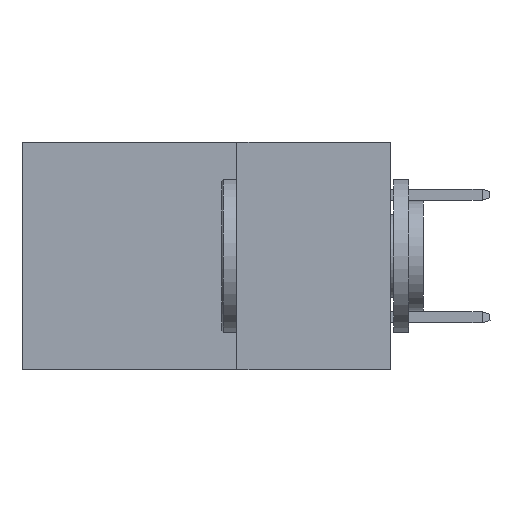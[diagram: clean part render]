
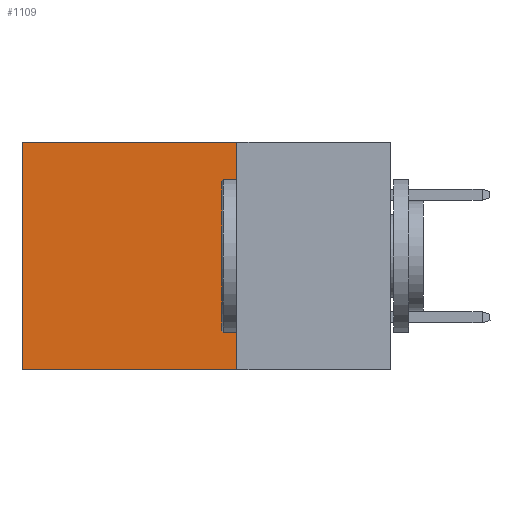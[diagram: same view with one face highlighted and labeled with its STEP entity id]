
A CAD part, left-side view. The second image highlights one B-rep face of the part: STEP entity #1109.
In plain terms, the highlighted planar face has unit normal (-1, 0, 0).
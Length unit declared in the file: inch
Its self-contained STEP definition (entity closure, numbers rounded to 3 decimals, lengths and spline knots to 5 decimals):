
#375 = EDGE_CURVE ( 'NONE', #5751, #5305, #4134, .T. ) ;
#1109 = ADVANCED_FACE ( 'NONE', ( #7847 ), #7928, .F. ) ;
#1123 = DIRECTION ( 'NONE',  ( 0., 0., -1. ) ) ;
#1485 = LINE ( 'NONE', #7017, #2935 ) ;
#1949 = ORIENTED_EDGE ( 'NONE', *, *, #10563, .F. ) ;
#2291 = LINE ( 'NONE', #9140, #10868 ) ;
#2491 = DIRECTION ( 'NONE',  ( 0., 1., 0. ) ) ;
#2551 = VECTOR ( 'NONE', #2491, 39.37008 ) ;
#2935 = VECTOR ( 'NONE', #5424, 39.37008 ) ;
#3433 = AXIS2_PLACEMENT_3D ( 'NONE', #3686, #5379, #1123 ) ;
#3471 = VERTEX_POINT ( 'NONE', #6926 ) ;
#3686 = CARTESIAN_POINT ( 'NONE',  ( 0.2875, 0.25, 0. ) ) ;
#4134 = LINE ( 'NONE', #4436, #5934 ) ;
#4308 = CARTESIAN_POINT ( 'NONE',  ( 0.2875, 0.25, -0.37 ) ) ;
#4430 = ORIENTED_EDGE ( 'NONE', *, *, #9543, .F. ) ;
#4436 = CARTESIAN_POINT ( 'NONE',  ( 0.2875, 0.25, 0. ) ) ;
#5018 = CARTESIAN_POINT ( 'NONE',  ( 0.2875, 0.6, -0.37 ) ) ;
#5305 = VERTEX_POINT ( 'NONE', #8914 ) ;
#5379 = DIRECTION ( 'NONE',  ( 1., 0., 0. ) ) ;
#5424 = DIRECTION ( 'NONE',  ( 0., 0., -1. ) ) ;
#5751 = VERTEX_POINT ( 'NONE', #9515 ) ;
#5788 = ORIENTED_EDGE ( 'NONE', *, *, #9982, .T. ) ;
#5934 = VECTOR ( 'NONE', #10287, 39.37008 ) ;
#6057 = EDGE_LOOP ( 'NONE', ( #5788, #1949, #4430, #7060 ) ) ;
#6926 = CARTESIAN_POINT ( 'NONE',  ( 0.2875, 0.25, -0.37 ) ) ;
#7017 = CARTESIAN_POINT ( 'NONE',  ( 0.2875, 0.6, 0. ) ) ;
#7060 = ORIENTED_EDGE ( 'NONE', *, *, #375, .T. ) ;
#7847 = FACE_OUTER_BOUND ( 'NONE', #6057, .T. ) ;
#7928 = PLANE ( 'NONE',  #3433 ) ;
#8914 = CARTESIAN_POINT ( 'NONE',  ( 0.2875, 0.6, 0. ) ) ;
#9073 = DIRECTION ( 'NONE',  ( 0., 0., -1. ) ) ;
#9140 = CARTESIAN_POINT ( 'NONE',  ( 0.2875, 0.25, 0. ) ) ;
#9147 = VERTEX_POINT ( 'NONE', #5018 ) ;
#9506 = LINE ( 'NONE', #4308, #2551 ) ;
#9515 = CARTESIAN_POINT ( 'NONE',  ( 0.2875, 0.25, 0. ) ) ;
#9543 = EDGE_CURVE ( 'NONE', #5751, #3471, #2291, .T. ) ;
#9982 = EDGE_CURVE ( 'NONE', #5305, #9147, #1485, .T. ) ;
#10287 = DIRECTION ( 'NONE',  ( 0., 1., 0. ) ) ;
#10563 = EDGE_CURVE ( 'NONE', #3471, #9147, #9506, .T. ) ;
#10868 = VECTOR ( 'NONE', #9073, 39.37008 ) ;
